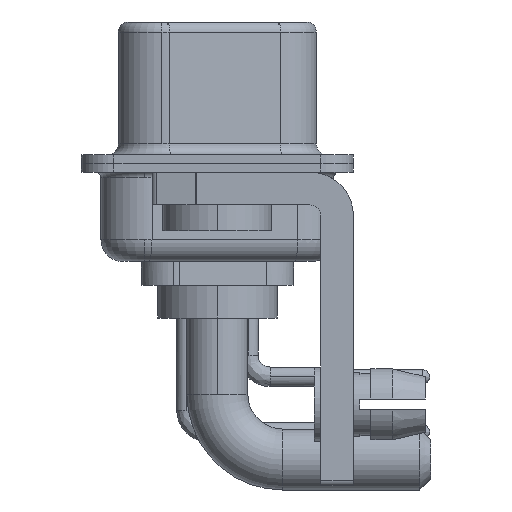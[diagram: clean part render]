
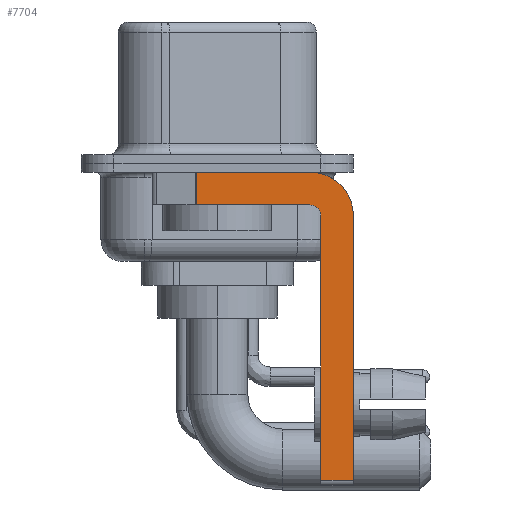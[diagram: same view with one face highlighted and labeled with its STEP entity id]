
A CAD part, left-side view. The second image highlights one B-rep face of the part: STEP entity #7704.
In plain terms, the highlighted planar face has unit normal (-1, 0, 0).
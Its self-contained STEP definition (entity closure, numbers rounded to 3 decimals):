
#79 = CIRCLE ( 'NONE', #28059, 2. ) ;
#536 = LINE ( 'NONE', #27713, #8459 ) ;
#821 = VERTEX_POINT ( 'NONE', #7438 ) ;
#1096 = LINE ( 'NONE', #25326, #3817 ) ;
#1164 = DIRECTION ( 'NONE',  ( 0., 0., 1. ) ) ;
#1516 = PLANE ( 'NONE',  #9036 ) ;
#2251 = VERTEX_POINT ( 'NONE', #15165 ) ;
#2513 = LINE ( 'NONE', #22417, #10014 ) ;
#3024 = ORIENTED_EDGE ( 'NONE', *, *, #9242, .F. ) ;
#3745 = FACE_OUTER_BOUND ( 'NONE', #11632, .T. ) ;
#3817 = VECTOR ( 'NONE', #5239, 1000. ) ;
#4199 = EDGE_CURVE ( 'NONE', #821, #2251, #19113, .T. ) ;
#4410 = VERTEX_POINT ( 'NONE', #13436 ) ;
#5239 = DIRECTION ( 'NONE',  ( 0., 1., 0. ) ) ;
#6191 = CARTESIAN_POINT ( 'NONE',  ( -2.9, 0.978, -1.9 ) ) ;
#6907 = LINE ( 'NONE', #29202, #21908 ) ;
#7245 = CARTESIAN_POINT ( 'NONE',  ( -2.9, -4.25, -1.9 ) ) ;
#7438 = CARTESIAN_POINT ( 'NONE',  ( -2.9, -4.75, -14.55 ) ) ;
#7704 = ADVANCED_FACE ( 'NONE', ( #3745 ), #1516, .F. ) ;
#7885 = EDGE_CURVE ( 'NONE', #2251, #21913, #17510, .T. ) ;
#8327 = DIRECTION ( 'NONE',  ( 0., 0., 1. ) ) ;
#8420 = CARTESIAN_POINT ( 'NONE',  ( -2.9, -4.25, -14.55 ) ) ;
#8459 = VECTOR ( 'NONE', #23258, 1000. ) ;
#9036 = AXIS2_PLACEMENT_3D ( 'NONE', #12187, #19473, #28529 ) ;
#9242 = EDGE_CURVE ( 'NONE', #21913, #20135, #1096, .T. ) ;
#9296 = DIRECTION ( 'NONE',  ( 1., 0., 0. ) ) ;
#9494 = ORIENTED_EDGE ( 'NONE', *, *, #4199, .F. ) ;
#9531 = CARTESIAN_POINT ( 'NONE',  ( -2.9, -6.25, -2.4 ) ) ;
#10014 = VECTOR ( 'NONE', #11538, 1000. ) ;
#10869 = AXIS2_PLACEMENT_3D ( 'NONE', #17832, #28692, #8327 ) ;
#11538 = DIRECTION ( 'NONE',  ( 0., 0., -1. ) ) ;
#11632 = EDGE_LOOP ( 'NONE', ( #14345, #22740, #3024, #21201, #9494, #15264, #17079, #15285 ) ) ;
#12187 = CARTESIAN_POINT ( 'NONE',  ( -2.9, -4.25, -2.4 ) ) ;
#12731 = LINE ( 'NONE', #8420, #21992 ) ;
#13436 = CARTESIAN_POINT ( 'NONE',  ( -2.9, -4.25, -0.4 ) ) ;
#14328 = CARTESIAN_POINT ( 'NONE',  ( -2.9, -4.25, -2.4 ) ) ;
#14345 = ORIENTED_EDGE ( 'NONE', *, *, #20990, .F. ) ;
#14772 = EDGE_CURVE ( 'NONE', #821, #25822, #12731, .T. ) ;
#15165 = CARTESIAN_POINT ( 'NONE',  ( -2.9, -4.75, -2.4 ) ) ;
#15264 = ORIENTED_EDGE ( 'NONE', *, *, #14772, .T. ) ;
#15285 = ORIENTED_EDGE ( 'NONE', *, *, #23781, .F. ) ;
#17079 = ORIENTED_EDGE ( 'NONE', *, *, #25805, .F. ) ;
#17510 = CIRCLE ( 'NONE', #10869, 0.5 ) ;
#17832 = CARTESIAN_POINT ( 'NONE',  ( -2.9, -4.25, -2.4 ) ) ;
#18346 = DIRECTION ( 'NONE',  ( 0., 0., -1. ) ) ;
#18492 = VERTEX_POINT ( 'NONE', #23456 ) ;
#19113 = LINE ( 'NONE', #26258, #26428 ) ;
#19473 = DIRECTION ( 'NONE',  ( 1., 0., 0. ) ) ;
#19580 = DIRECTION ( 'NONE',  ( 0., -1., 0. ) ) ;
#20135 = VERTEX_POINT ( 'NONE', #6191 ) ;
#20619 = CARTESIAN_POINT ( 'NONE',  ( -2.9, -6.25, -14.55 ) ) ;
#20990 = EDGE_CURVE ( 'NONE', #18492, #4410, #536, .T. ) ;
#21201 = ORIENTED_EDGE ( 'NONE', *, *, #7885, .F. ) ;
#21908 = VECTOR ( 'NONE', #25065, 1000. ) ;
#21913 = VERTEX_POINT ( 'NONE', #7245 ) ;
#21992 = VECTOR ( 'NONE', #19580, 1000. ) ;
#22417 = CARTESIAN_POINT ( 'NONE',  ( -2.9, -6.25, -2.4 ) ) ;
#22740 = ORIENTED_EDGE ( 'NONE', *, *, #27673, .T. ) ;
#23258 = DIRECTION ( 'NONE',  ( 0., -1., 0. ) ) ;
#23456 = CARTESIAN_POINT ( 'NONE',  ( -2.9, 0.978, -0.4 ) ) ;
#23781 = EDGE_CURVE ( 'NONE', #4410, #28266, #79, .T. ) ;
#25065 = DIRECTION ( 'NONE',  ( 0., 0., -1. ) ) ;
#25326 = CARTESIAN_POINT ( 'NONE',  ( -2.9, -4.25, -1.9 ) ) ;
#25805 = EDGE_CURVE ( 'NONE', #28266, #25822, #2513, .T. ) ;
#25822 = VERTEX_POINT ( 'NONE', #20619 ) ;
#26258 = CARTESIAN_POINT ( 'NONE',  ( -2.9, -4.75, -14.8 ) ) ;
#26428 = VECTOR ( 'NONE', #1164, 1000. ) ;
#27673 = EDGE_CURVE ( 'NONE', #18492, #20135, #6907, .T. ) ;
#27713 = CARTESIAN_POINT ( 'NONE',  ( -2.9, 3., -0.4 ) ) ;
#28059 = AXIS2_PLACEMENT_3D ( 'NONE', #14328, #9296, #18346 ) ;
#28266 = VERTEX_POINT ( 'NONE', #9531 ) ;
#28529 = DIRECTION ( 'NONE',  ( 0., 0., -1. ) ) ;
#28692 = DIRECTION ( 'NONE',  ( -1., 0., 0. ) ) ;
#29202 = CARTESIAN_POINT ( 'NONE',  ( -2.9, 0.978, -1.9 ) ) ;
